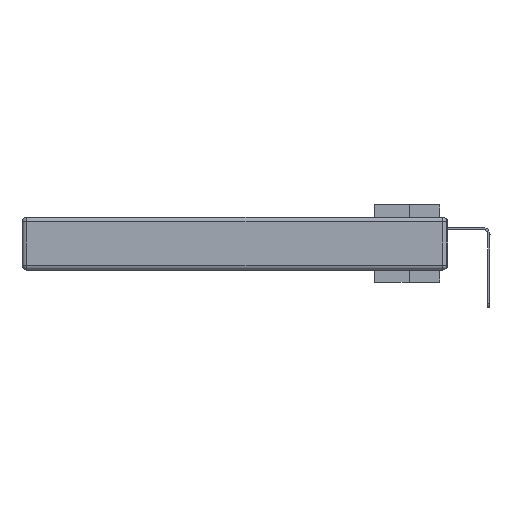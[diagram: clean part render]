
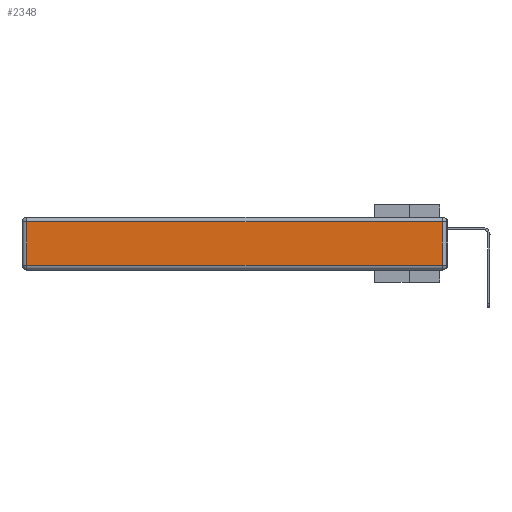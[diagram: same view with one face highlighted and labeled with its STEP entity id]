
A CAD part, left-side view. The second image highlights one B-rep face of the part: STEP entity #2348.
In plain terms, the highlighted planar face has unit normal (-1, 0, 0).
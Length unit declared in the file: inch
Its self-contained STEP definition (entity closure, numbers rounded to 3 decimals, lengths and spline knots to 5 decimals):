
#1040 = CARTESIAN_POINT ( 'NONE',  ( 0., 0.03, -0.313 ) ) ;
#2348 = ADVANCED_FACE ( 'NONE', ( #23503 ), #11074, .T. ) ;
#2970 = DIRECTION ( 'NONE',  ( 0., 0., -1. ) ) ;
#3099 = AXIS2_PLACEMENT_3D ( 'NONE', #36631, #13906, #11323 ) ;
#3773 = DIRECTION ( 'NONE',  ( 0., 0., 1. ) ) ;
#4149 = VECTOR ( 'NONE', #3773, 39.37008 ) ;
#4472 = VECTOR ( 'NONE', #13725, 39.37008 ) ;
#7487 = ORIENTED_EDGE ( 'NONE', *, *, #34548, .T. ) ;
#8503 = VECTOR ( 'NONE', #20744, 39.37008 ) ;
#8528 = CARTESIAN_POINT ( 'NONE',  ( 0., 2.72, -0.03 ) ) ;
#10082 = VERTEX_POINT ( 'NONE', #19275 ) ;
#11074 = PLANE ( 'NONE',  #3099 ) ;
#11323 = DIRECTION ( 'NONE',  ( 0., 0., 1. ) ) ;
#12650 = VERTEX_POINT ( 'NONE', #8528 ) ;
#13177 = LINE ( 'NONE', #20105, #34838 ) ;
#13725 = DIRECTION ( 'NONE',  ( 0., 1., 0. ) ) ;
#13906 = DIRECTION ( 'NONE',  ( -1., 0., 0. ) ) ;
#15329 = CARTESIAN_POINT ( 'NONE',  ( 0., 0.03, -0.343 ) ) ;
#16918 = LINE ( 'NONE', #28061, #4472 ) ;
#17388 = EDGE_CURVE ( 'NONE', #10082, #30214, #26274, .T. ) ;
#17921 = CARTESIAN_POINT ( 'NONE',  ( 0., 0., -0.313 ) ) ;
#19275 = CARTESIAN_POINT ( 'NONE',  ( 0., 2.72, -0.313 ) ) ;
#20105 = CARTESIAN_POINT ( 'NONE',  ( 0., 2.72, -0.343 ) ) ;
#20440 = ORIENTED_EDGE ( 'NONE', *, *, #25686, .T. ) ;
#20744 = DIRECTION ( 'NONE',  ( 0., -1., 0. ) ) ;
#21435 = VERTEX_POINT ( 'NONE', #33591 ) ;
#22331 = LINE ( 'NONE', #15329, #4149 ) ;
#23503 = FACE_OUTER_BOUND ( 'NONE', #29259, .T. ) ;
#25686 = EDGE_CURVE ( 'NONE', #30214, #21435, #22331, .T. ) ;
#26274 = LINE ( 'NONE', #17921, #8503 ) ;
#26547 = ORIENTED_EDGE ( 'NONE', *, *, #17388, .T. ) ;
#28061 = CARTESIAN_POINT ( 'NONE',  ( 0., 2.75, -0.03 ) ) ;
#29259 = EDGE_LOOP ( 'NONE', ( #26547, #20440, #7487, #34725 ) ) ;
#29509 = EDGE_CURVE ( 'NONE', #12650, #10082, #13177, .T. ) ;
#30214 = VERTEX_POINT ( 'NONE', #1040 ) ;
#33591 = CARTESIAN_POINT ( 'NONE',  ( 0., 0.03, -0.03 ) ) ;
#34548 = EDGE_CURVE ( 'NONE', #21435, #12650, #16918, .T. ) ;
#34725 = ORIENTED_EDGE ( 'NONE', *, *, #29509, .T. ) ;
#34838 = VECTOR ( 'NONE', #2970, 39.37008 ) ;
#36631 = CARTESIAN_POINT ( 'NONE',  ( 0., 0., -0.343 ) ) ;
